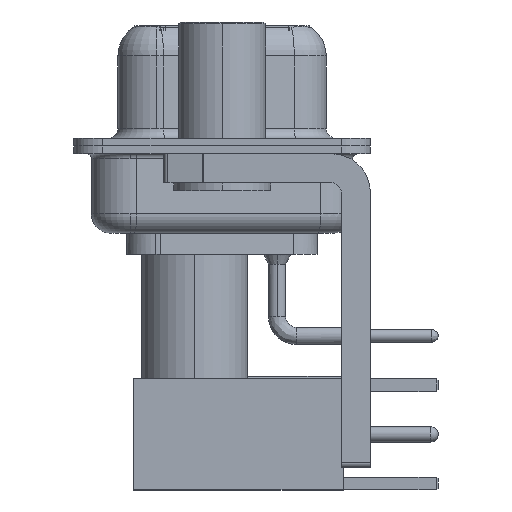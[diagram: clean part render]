
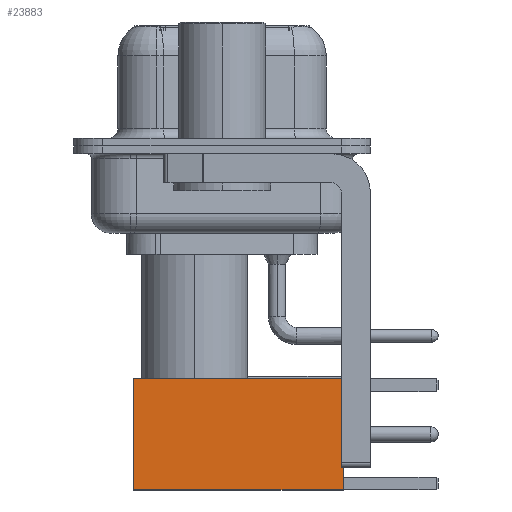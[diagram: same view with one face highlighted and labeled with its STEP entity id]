
A CAD part, left-side view. The second image highlights one B-rep face of the part: STEP entity #23883.
In plain terms, the highlighted face is planar.
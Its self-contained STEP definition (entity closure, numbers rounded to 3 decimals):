
#25 = VECTOR ( 'NONE', #4304, 1000. ) ;
#541 = VECTOR ( 'NONE', #16422, 1000. ) ;
#1699 = VERTEX_POINT ( 'NONE', #15322 ) ;
#2180 = VECTOR ( 'NONE', #10550, 1000. ) ;
#2823 = CARTESIAN_POINT ( 'NONE',  ( 2.875, 2.875, 0. ) ) ;
#4304 = DIRECTION ( 'NONE',  ( 0., 0., -1. ) ) ;
#4403 = AXIS2_PLACEMENT_3D ( 'NONE', #2823, #5356, #16966 ) ;
#4432 = DIRECTION ( 'NONE',  ( 0., 0., -1. ) ) ;
#5352 = LINE ( 'NONE', #5894, #541 ) ;
#5356 = DIRECTION ( 'NONE',  ( 0., 1., 0. ) ) ;
#5419 = ORIENTED_EDGE ( 'NONE', *, *, #28450, .F. ) ;
#5894 = CARTESIAN_POINT ( 'NONE',  ( 0., 2.875, 10.82 ) ) ;
#5902 = EDGE_CURVE ( 'NONE', #12325, #1699, #31677, .T. ) ;
#8619 = PLANE ( 'NONE',  #4403 ) ;
#8748 = ORIENTED_EDGE ( 'NONE', *, *, #5902, .T. ) ;
#9509 = ORIENTED_EDGE ( 'NONE', *, *, #28732, .F. ) ;
#10550 = DIRECTION ( 'NONE',  ( -1., 0., 0. ) ) ;
#12325 = VERTEX_POINT ( 'NONE', #24117 ) ;
#15322 = CARTESIAN_POINT ( 'NONE',  ( 2.875, 2.875, 0. ) ) ;
#15364 = VERTEX_POINT ( 'NONE', #25710 ) ;
#16422 = DIRECTION ( 'NONE',  ( -1., 0., 0. ) ) ;
#16966 = DIRECTION ( 'NONE',  ( 0., 0., 1. ) ) ;
#18692 = LINE ( 'NONE', #29736, #2180 ) ;
#20679 = VERTEX_POINT ( 'NONE', #33355 ) ;
#21077 = EDGE_LOOP ( 'NONE', ( #8748, #22920, #9509, #5419 ) ) ;
#22920 = ORIENTED_EDGE ( 'NONE', *, *, #32059, .T. ) ;
#23883 = ADVANCED_FACE ( 'NONE', ( #33452 ), #8619, .T. ) ;
#24117 = CARTESIAN_POINT ( 'NONE',  ( 2.875, 2.875, 10.82 ) ) ;
#25710 = CARTESIAN_POINT ( 'NONE',  ( -2.875, 2.875, 10.82 ) ) ;
#26720 = CARTESIAN_POINT ( 'NONE',  ( -2.875, 2.875, 0. ) ) ;
#27075 = LINE ( 'NONE', #26720, #30678 ) ;
#28450 = EDGE_CURVE ( 'NONE', #12325, #15364, #5352, .T. ) ;
#28732 = EDGE_CURVE ( 'NONE', #15364, #20679, #27075, .T. ) ;
#29136 = CARTESIAN_POINT ( 'NONE',  ( 2.875, 2.875, 0. ) ) ;
#29736 = CARTESIAN_POINT ( 'NONE',  ( 0., 2.875, 0. ) ) ;
#30678 = VECTOR ( 'NONE', #4432, 1000. ) ;
#31677 = LINE ( 'NONE', #29136, #25 ) ;
#32059 = EDGE_CURVE ( 'NONE', #1699, #20679, #18692, .T. ) ;
#33355 = CARTESIAN_POINT ( 'NONE',  ( -2.875, 2.875, 0. ) ) ;
#33452 = FACE_OUTER_BOUND ( 'NONE', #21077, .T. ) ;
